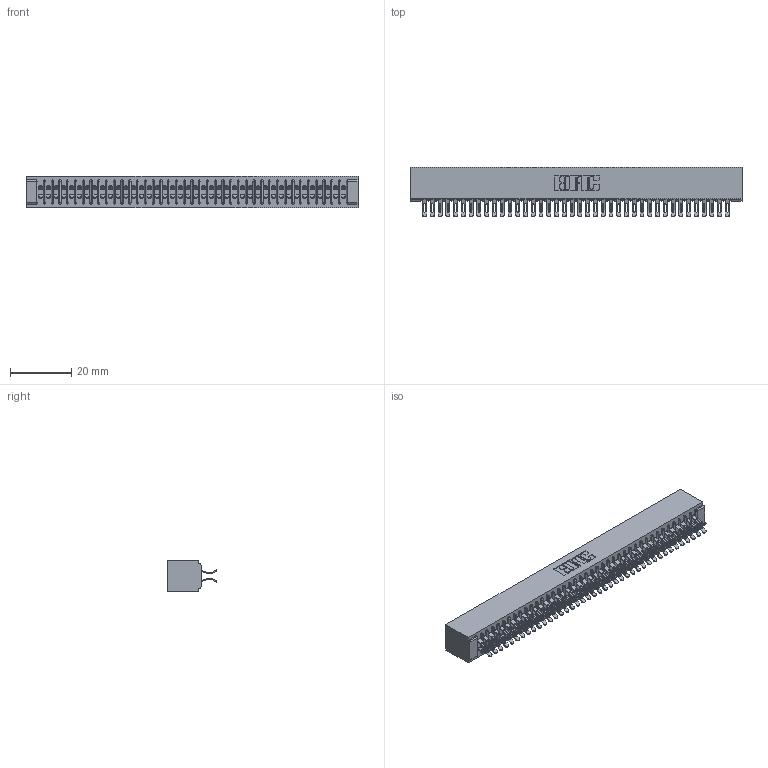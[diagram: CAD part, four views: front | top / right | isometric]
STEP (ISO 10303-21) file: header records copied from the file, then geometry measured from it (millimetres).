
FILE_DESCRIPTION (( 'STEP AP203' ), '1' );
FILE_NAME ('341-080-555-201.STEP', '2018-08-07T21:48:01', ( '' ), ( '' ), 'SwSTEP 2.0', 'SolidWorks 2016', '' );
FILE_SCHEMA (( 'CONFIG_CONTROL_DESIGN' ));
Length unit declared in the file: inch
Products named in the file (3): 341 Part_No Mounting Lugs; 341-292-001_341-292-155; 341-080-555-201
Assembly tree (81 placements, depth 2):
  341-080-555-201
    341 Part_No Mounting Lugs
    341-292-001_341-292-155  x80
Bounding box: 108.58 x 16.31 x 10.16 mm (x, y, z)
Volume: 8354.2 mm3; surface area: 16081.8 mm2
Topology: 81 solids, 81 shells, 6348 faces, 18972 edges, 12350 vertices
Faces by surface type: plane 3424, cylinder 2764, sphere 82, torus 78
Entity records: 48867 total; most frequent: CARTESIAN_POINT 8138, ORIENTED_EDGE 8076, DIRECTION 7888, EDGE_CURVE 4038, LINE 3248, VECTOR 3248, VERTEX_POINT 2554, AXIS2_PLACEMENT_3D 2320
